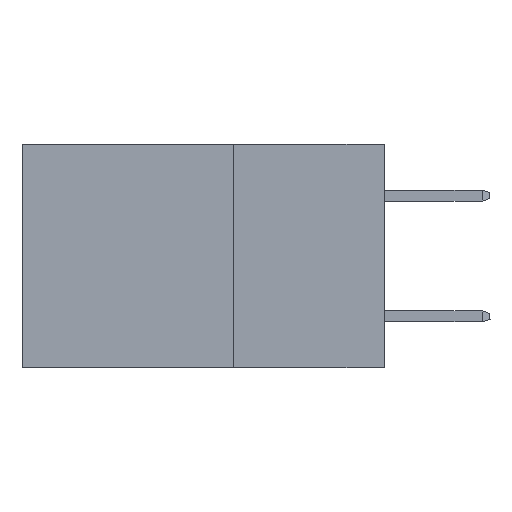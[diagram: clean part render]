
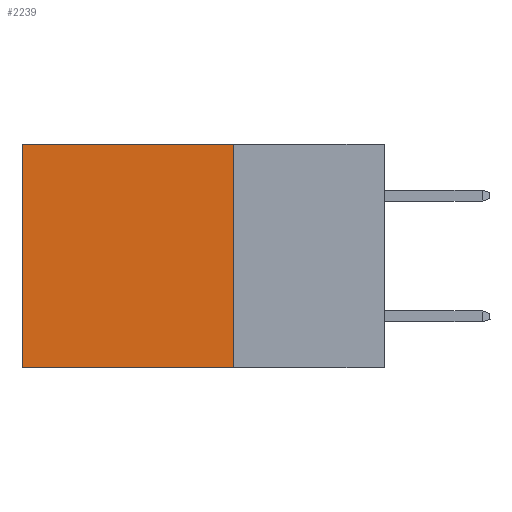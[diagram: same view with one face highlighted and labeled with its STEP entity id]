
A CAD part, left-side view. The second image highlights one B-rep face of the part: STEP entity #2239.
In plain terms, the highlighted planar face has unit normal (-1, 0, 0).
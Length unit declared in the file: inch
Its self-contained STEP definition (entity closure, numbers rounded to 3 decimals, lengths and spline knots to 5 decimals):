
#76 = AXIS2_PLACEMENT_3D ( 'NONE', #21458, #17721, #16572 ) ;
#173 = VERTEX_POINT ( 'NONE', #7327 ) ;
#1066 = CARTESIAN_POINT ( 'NONE',  ( 0.2615, 0.25, -0.37 ) ) ;
#1293 = VECTOR ( 'NONE', #19991, 39.37008 ) ;
#1524 = EDGE_LOOP ( 'NONE', ( #6821, #13868, #21735, #21306 ) ) ;
#2239 = ADVANCED_FACE ( 'NONE', ( #13032 ), #7999, .F. ) ;
#6759 = EDGE_CURVE ( 'NONE', #13223, #6952, #15599, .T. ) ;
#6798 = LINE ( 'NONE', #15951, #1293 ) ;
#6821 = ORIENTED_EDGE ( 'NONE', *, *, #18621, .T. ) ;
#6952 = VERTEX_POINT ( 'NONE', #19470 ) ;
#7327 = CARTESIAN_POINT ( 'NONE',  ( 0.2615, 0.25, -0.37 ) ) ;
#7999 = PLANE ( 'NONE',  #76 ) ;
#9331 = DIRECTION ( 'NONE',  ( 0., 0., -1. ) ) ;
#9626 = LINE ( 'NONE', #1066, #19599 ) ;
#10282 = CARTESIAN_POINT ( 'NONE',  ( 0.2615, 0.6, -0.37 ) ) ;
#10355 = VECTOR ( 'NONE', #18951, 39.37008 ) ;
#10756 = VERTEX_POINT ( 'NONE', #10282 ) ;
#13032 = FACE_OUTER_BOUND ( 'NONE', #1524, .T. ) ;
#13176 = CARTESIAN_POINT ( 'NONE',  ( 0.2615, 0.25, 0. ) ) ;
#13223 = VERTEX_POINT ( 'NONE', #13176 ) ;
#13868 = ORIENTED_EDGE ( 'NONE', *, *, #20972, .F. ) ;
#15599 = LINE ( 'NONE', #16941, #10355 ) ;
#15951 = CARTESIAN_POINT ( 'NONE',  ( 0.2615, 0.6, -0.37 ) ) ;
#16572 = DIRECTION ( 'NONE',  ( 0., 0., -1. ) ) ;
#16941 = CARTESIAN_POINT ( 'NONE',  ( 0.2615, 0.25, 0. ) ) ;
#17721 = DIRECTION ( 'NONE',  ( 1., 0., 0. ) ) ;
#18621 = EDGE_CURVE ( 'NONE', #6952, #10756, #6798, .T. ) ;
#18951 = DIRECTION ( 'NONE',  ( 0., 1., 0. ) ) ;
#19470 = CARTESIAN_POINT ( 'NONE',  ( 0.2615, 0.6, 0. ) ) ;
#19599 = VECTOR ( 'NONE', #9331, 39.37008 ) ;
#19991 = DIRECTION ( 'NONE',  ( 0., 0., -1. ) ) ;
#20972 = EDGE_CURVE ( 'NONE', #173, #10756, #24688, .T. ) ;
#21306 = ORIENTED_EDGE ( 'NONE', *, *, #6759, .T. ) ;
#21458 = CARTESIAN_POINT ( 'NONE',  ( 0.2615, 0.25, -0.37 ) ) ;
#21735 = ORIENTED_EDGE ( 'NONE', *, *, #22513, .F. ) ;
#22043 = CARTESIAN_POINT ( 'NONE',  ( 0.2615, 0.25, -0.37 ) ) ;
#22513 = EDGE_CURVE ( 'NONE', #13223, #173, #9626, .T. ) ;
#24053 = VECTOR ( 'NONE', #26049, 39.37008 ) ;
#24688 = LINE ( 'NONE', #22043, #24053 ) ;
#26049 = DIRECTION ( 'NONE',  ( 0., 1., 0. ) ) ;
